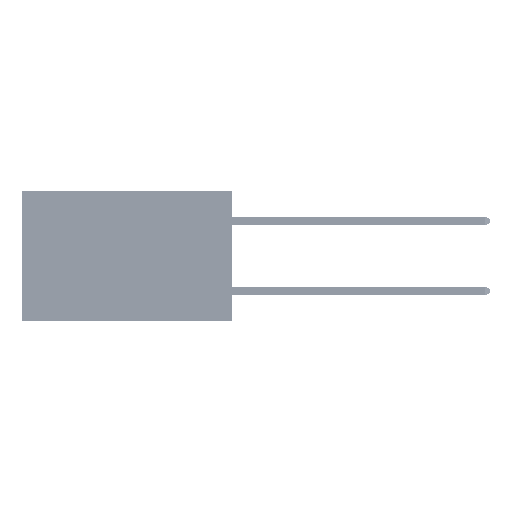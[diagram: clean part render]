
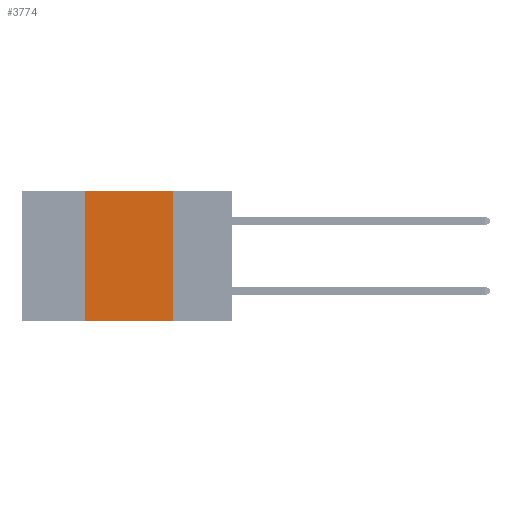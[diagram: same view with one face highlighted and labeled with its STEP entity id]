
A CAD part, left-side view. The second image highlights one B-rep face of the part: STEP entity #3774.
In plain terms, the highlighted planar face has unit normal (-1, 0, 0).
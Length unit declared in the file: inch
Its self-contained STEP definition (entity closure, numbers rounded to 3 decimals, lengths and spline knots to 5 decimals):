
#81 = DIRECTION ( 'NONE',  ( 0., 0., -1. ) ) ;
#319 = CARTESIAN_POINT ( 'NONE',  ( 0., 0.42, 0. ) ) ;
#525 = DIRECTION ( 'NONE',  ( 0., 0., -1. ) ) ;
#3689 = VECTOR ( 'NONE', #35626, 39.37008 ) ;
#3774 = ADVANCED_FACE ( 'NONE', ( #5073 ), #25743, .F. ) ;
#5073 = FACE_OUTER_BOUND ( 'NONE', #17346, .T. ) ;
#6248 = LINE ( 'NONE', #50561, #44369 ) ;
#7810 = LINE ( 'NONE', #16131, #48355 ) ;
#9640 = CARTESIAN_POINT ( 'NONE',  ( 0., 0.6, 0. ) ) ;
#11900 = CARTESIAN_POINT ( 'NONE',  ( 0., 0.17, 0. ) ) ;
#12120 = VECTOR ( 'NONE', #81, 39.37008 ) ;
#13756 = VERTEX_POINT ( 'NONE', #319 ) ;
#14547 = DIRECTION ( 'NONE',  ( 0., 0., 1. ) ) ;
#15603 = DIRECTION ( 'NONE',  ( 0., -1., 0. ) ) ;
#16131 = CARTESIAN_POINT ( 'NONE',  ( 0., 0.6, -0.37 ) ) ;
#17346 = EDGE_LOOP ( 'NONE', ( #52089, #29166, #27777, #33938 ) ) ;
#17779 = CARTESIAN_POINT ( 'NONE',  ( 0., 0.17, 0. ) ) ;
#20932 = VERTEX_POINT ( 'NONE', #25718 ) ;
#21167 = EDGE_CURVE ( 'NONE', #13756, #38182, #44216, .T. ) ;
#25718 = CARTESIAN_POINT ( 'NONE',  ( 0., 0.42, -0.37 ) ) ;
#25743 = PLANE ( 'NONE',  #35430 ) ;
#27777 = ORIENTED_EDGE ( 'NONE', *, *, #28929, .F. ) ;
#28929 = EDGE_CURVE ( 'NONE', #20932, #13756, #6248, .T. ) ;
#29166 = ORIENTED_EDGE ( 'NONE', *, *, #21167, .F. ) ;
#32416 = CARTESIAN_POINT ( 'NONE',  ( 0., 0.17, -0.37 ) ) ;
#33938 = ORIENTED_EDGE ( 'NONE', *, *, #40453, .T. ) ;
#35430 = AXIS2_PLACEMENT_3D ( 'NONE', #9640, #46154, #525 ) ;
#35626 = DIRECTION ( 'NONE',  ( 0., -1., 0. ) ) ;
#37992 = EDGE_CURVE ( 'NONE', #38182, #38942, #40347, .T. ) ;
#38182 = VERTEX_POINT ( 'NONE', #17779 ) ;
#38942 = VERTEX_POINT ( 'NONE', #32416 ) ;
#40347 = LINE ( 'NONE', #11900, #12120 ) ;
#40453 = EDGE_CURVE ( 'NONE', #20932, #38942, #7810, .T. ) ;
#44216 = LINE ( 'NONE', #44750, #3689 ) ;
#44369 = VECTOR ( 'NONE', #14547, 39.37008 ) ;
#44750 = CARTESIAN_POINT ( 'NONE',  ( 0., 0.6, 0. ) ) ;
#46154 = DIRECTION ( 'NONE',  ( 1., 0., 0. ) ) ;
#48355 = VECTOR ( 'NONE', #15603, 39.37008 ) ;
#50561 = CARTESIAN_POINT ( 'NONE',  ( 0., 0.42, 0. ) ) ;
#52089 = ORIENTED_EDGE ( 'NONE', *, *, #37992, .F. ) ;
